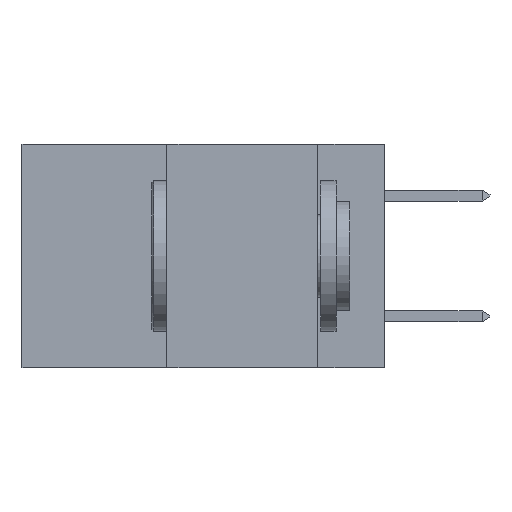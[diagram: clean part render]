
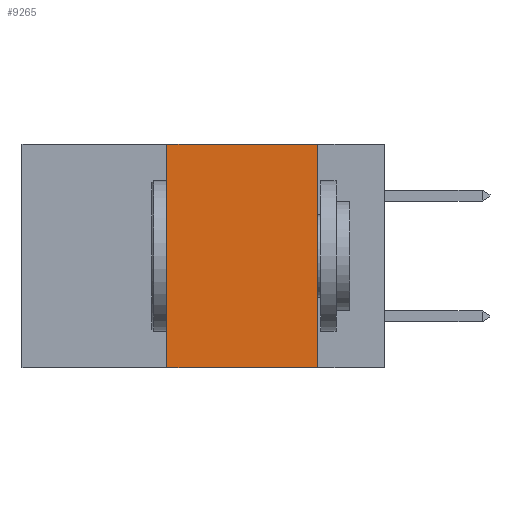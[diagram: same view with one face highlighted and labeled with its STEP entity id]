
A CAD part, left-side view. The second image highlights one B-rep face of the part: STEP entity #9265.
In plain terms, the highlighted planar face has unit normal (-1, 0, 0).
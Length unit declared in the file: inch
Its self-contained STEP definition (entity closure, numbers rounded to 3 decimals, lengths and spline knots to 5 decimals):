
#169 = VERTEX_POINT ( 'NONE', #13486 ) ;
#1014 = CARTESIAN_POINT ( 'NONE',  ( 0., 0.11, -0.37 ) ) ;
#1572 = VERTEX_POINT ( 'NONE', #9802 ) ;
#3387 = VERTEX_POINT ( 'NONE', #18475 ) ;
#4080 = DIRECTION ( 'NONE',  ( 0., -1., 0. ) ) ;
#6272 = ORIENTED_EDGE ( 'NONE', *, *, #8924, .T. ) ;
#6339 = EDGE_CURVE ( 'NONE', #1572, #20094, #18012, .T. ) ;
#7325 = VECTOR ( 'NONE', #7939, 39.37008 ) ;
#7772 = PLANE ( 'NONE',  #11615 ) ;
#7853 = DIRECTION ( 'NONE',  ( 0., 0., -1. ) ) ;
#7939 = DIRECTION ( 'NONE',  ( 0., 0., -1. ) ) ;
#8088 = ORIENTED_EDGE ( 'NONE', *, *, #23127, .F. ) ;
#8924 = EDGE_CURVE ( 'NONE', #3387, #20094, #17219, .T. ) ;
#9265 = ADVANCED_FACE ( 'NONE', ( #11667 ), #7772, .F. ) ;
#9730 = EDGE_LOOP ( 'NONE', ( #22581, #16551, #8088, #6272 ) ) ;
#9802 = CARTESIAN_POINT ( 'NONE',  ( 0., 0.11, 0. ) ) ;
#9889 = LINE ( 'NONE', #11870, #19078 ) ;
#9913 = DIRECTION ( 'NONE',  ( 1., 0., 0. ) ) ;
#10362 = DIRECTION ( 'NONE',  ( 0., -1., 0. ) ) ;
#10599 = CARTESIAN_POINT ( 'NONE',  ( 0., 0.6, -0.37 ) ) ;
#11615 = AXIS2_PLACEMENT_3D ( 'NONE', #19595, #9913, #7853 ) ;
#11667 = FACE_OUTER_BOUND ( 'NONE', #9730, .T. ) ;
#11870 = CARTESIAN_POINT ( 'NONE',  ( 0., 0.6, 0. ) ) ;
#13486 = CARTESIAN_POINT ( 'NONE',  ( 0., 0.36, 0. ) ) ;
#13785 = EDGE_CURVE ( 'NONE', #169, #1572, #9889, .T. ) ;
#16551 = ORIENTED_EDGE ( 'NONE', *, *, #13785, .F. ) ;
#17219 = LINE ( 'NONE', #10599, #21192 ) ;
#18012 = LINE ( 'NONE', #21888, #7325 ) ;
#18475 = CARTESIAN_POINT ( 'NONE',  ( 0., 0.36, -0.37 ) ) ;
#19078 = VECTOR ( 'NONE', #4080, 39.37008 ) ;
#19595 = CARTESIAN_POINT ( 'NONE',  ( 0., 0.6, 0. ) ) ;
#19887 = VECTOR ( 'NONE', #24668, 39.37008 ) ;
#20094 = VERTEX_POINT ( 'NONE', #1014 ) ;
#21192 = VECTOR ( 'NONE', #10362, 39.37008 ) ;
#21888 = CARTESIAN_POINT ( 'NONE',  ( 0., 0.11, 0. ) ) ;
#22027 = LINE ( 'NONE', #24845, #19887 ) ;
#22581 = ORIENTED_EDGE ( 'NONE', *, *, #6339, .F. ) ;
#23127 = EDGE_CURVE ( 'NONE', #3387, #169, #22027, .T. ) ;
#24668 = DIRECTION ( 'NONE',  ( 0., 0., 1. ) ) ;
#24845 = CARTESIAN_POINT ( 'NONE',  ( 0., 0.36, 0. ) ) ;
